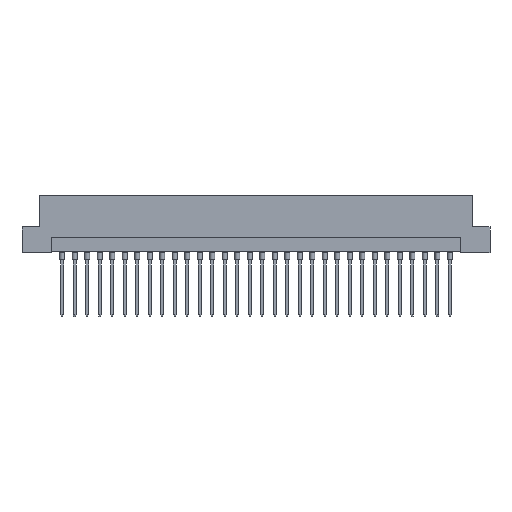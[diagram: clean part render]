
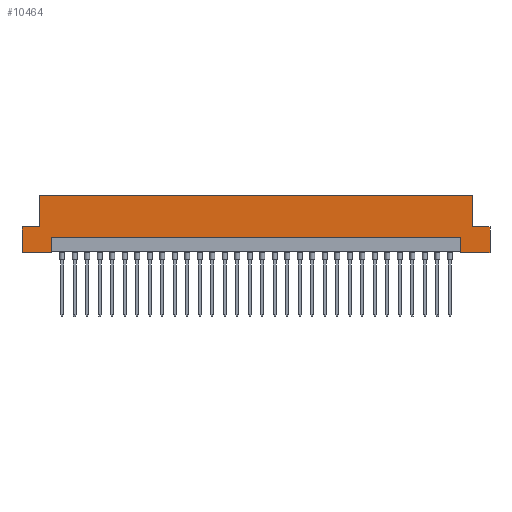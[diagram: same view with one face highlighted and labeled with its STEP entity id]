
A CAD part, front view. The second image highlights one B-rep face of the part: STEP entity #10464.
In plain terms, the highlighted planar face has unit normal (0, -1, 0).
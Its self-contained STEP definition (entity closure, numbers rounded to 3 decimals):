
#537 = CARTESIAN_POINT ( 'NONE',  ( -41.6, -4.3, 0. ) ) ;
#689 = ORIENTED_EDGE ( 'NONE', *, *, #5636, .F. ) ;
#698 = EDGE_CURVE ( 'NONE', #7802, #4916, #2948, .T. ) ;
#783 = DIRECTION ( 'NONE',  ( 1., 0., 0. ) ) ;
#962 = LINE ( 'NONE', #6274, #11961 ) ;
#1484 = ORIENTED_EDGE ( 'NONE', *, *, #698, .F. ) ;
#1489 = VECTOR ( 'NONE', #2459, 1000. ) ;
#1511 = VECTOR ( 'NONE', #783, 1000. ) ;
#1996 = CARTESIAN_POINT ( 'NONE',  ( 47.5, -4.3, 0. ) ) ;
#2158 = DIRECTION ( 'NONE',  ( 1., 0., 0. ) ) ;
#2159 = EDGE_CURVE ( 'NONE', #3640, #11440, #4019, .T. ) ;
#2447 = VECTOR ( 'NONE', #13092, 1000. ) ;
#2459 = DIRECTION ( 'NONE',  ( 1., 0., 0. ) ) ;
#2513 = LINE ( 'NONE', #3584, #10403 ) ;
#2587 = VECTOR ( 'NONE', #7142, 1000. ) ;
#2603 = LINE ( 'NONE', #9913, #11557 ) ;
#2709 = ORIENTED_EDGE ( 'NONE', *, *, #9408, .T. ) ;
#2948 = LINE ( 'NONE', #4141, #6473 ) ;
#3002 = CARTESIAN_POINT ( 'NONE',  ( -47.5, -4.3, 5.2 ) ) ;
#3094 = DIRECTION ( 'NONE',  ( 0., 0., -1. ) ) ;
#3239 = ORIENTED_EDGE ( 'NONE', *, *, #9156, .F. ) ;
#3276 = EDGE_CURVE ( 'NONE', #5323, #5963, #2603, .T. ) ;
#3437 = CARTESIAN_POINT ( 'NONE',  ( 41.6, -4.3, 0. ) ) ;
#3564 = EDGE_CURVE ( 'NONE', #6624, #9732, #5309, .T. ) ;
#3584 = CARTESIAN_POINT ( 'NONE',  ( 41.6, -4.3, 0.2 ) ) ;
#3640 = VERTEX_POINT ( 'NONE', #3437 ) ;
#3717 = CARTESIAN_POINT ( 'NONE',  ( 47.5, -4.3, 11.6 ) ) ;
#3839 = ORIENTED_EDGE ( 'NONE', *, *, #3902, .T. ) ;
#3902 = EDGE_CURVE ( 'NONE', #11890, #5963, #6824, .T. ) ;
#3930 = CARTESIAN_POINT ( 'NONE',  ( 47.5, -4.3, 5.2 ) ) ;
#4019 = LINE ( 'NONE', #11302, #8169 ) ;
#4032 = DIRECTION ( 'NONE',  ( -1., 0., 0. ) ) ;
#4141 = CARTESIAN_POINT ( 'NONE',  ( -44., -4.3, 5.2 ) ) ;
#4298 = ORIENTED_EDGE ( 'NONE', *, *, #5062, .F. ) ;
#4318 = CARTESIAN_POINT ( 'NONE',  ( 47.5, -4.3, 11.6 ) ) ;
#4456 = VECTOR ( 'NONE', #2158, 1000. ) ;
#4537 = AXIS2_PLACEMENT_3D ( 'NONE', #3717, #6079, #4032 ) ;
#4629 = CARTESIAN_POINT ( 'NONE',  ( 41.6, -4.3, 3. ) ) ;
#4786 = EDGE_CURVE ( 'NONE', #5323, #8736, #12894, .T. ) ;
#4810 = LINE ( 'NONE', #8719, #12596 ) ;
#4916 = VERTEX_POINT ( 'NONE', #7189 ) ;
#4926 = VERTEX_POINT ( 'NONE', #3002 ) ;
#5013 = CARTESIAN_POINT ( 'NONE',  ( 44., -4.3, 5.2 ) ) ;
#5062 = EDGE_CURVE ( 'NONE', #4916, #9787, #8495, .T. ) ;
#5309 = LINE ( 'NONE', #3930, #2447 ) ;
#5323 = VERTEX_POINT ( 'NONE', #13076 ) ;
#5636 = EDGE_CURVE ( 'NONE', #3640, #8736, #2513, .T. ) ;
#5833 = EDGE_CURVE ( 'NONE', #4926, #7802, #9187, .T. ) ;
#5963 = VERTEX_POINT ( 'NONE', #537 ) ;
#6079 = DIRECTION ( 'NONE',  ( 0., 1., 0. ) ) ;
#6274 = CARTESIAN_POINT ( 'NONE',  ( 47.5, -4.3, 11.6 ) ) ;
#6473 = VECTOR ( 'NONE', #11171, 1000. ) ;
#6521 = CARTESIAN_POINT ( 'NONE',  ( 44., -4.3, 11.6 ) ) ;
#6624 = VERTEX_POINT ( 'NONE', #7639 ) ;
#6824 = LINE ( 'NONE', #10874, #1511 ) ;
#6860 = CARTESIAN_POINT ( 'NONE',  ( -41.6, -4.3, 3. ) ) ;
#7142 = DIRECTION ( 'NONE',  ( 0., 0., 1. ) ) ;
#7189 = CARTESIAN_POINT ( 'NONE',  ( -44., -4.3, 11.6 ) ) ;
#7532 = ORIENTED_EDGE ( 'NONE', *, *, #2159, .T. ) ;
#7557 = EDGE_CURVE ( 'NONE', #6624, #9787, #8068, .T. ) ;
#7623 = DIRECTION ( 'NONE',  ( 0., 0., 1. ) ) ;
#7639 = CARTESIAN_POINT ( 'NONE',  ( 44., -4.3, 5.2 ) ) ;
#7649 = DIRECTION ( 'NONE',  ( 0., 0., -1. ) ) ;
#7802 = VERTEX_POINT ( 'NONE', #12959 ) ;
#8060 = DIRECTION ( 'NONE',  ( 1., 0., 0. ) ) ;
#8068 = LINE ( 'NONE', #5013, #2587 ) ;
#8169 = VECTOR ( 'NONE', #8060, 1000. ) ;
#8199 = CARTESIAN_POINT ( 'NONE',  ( -47.5, -4.3, 5.2 ) ) ;
#8495 = LINE ( 'NONE', #4318, #1489 ) ;
#8719 = CARTESIAN_POINT ( 'NONE',  ( -47.5, -4.3, 11.6 ) ) ;
#8736 = VERTEX_POINT ( 'NONE', #4629 ) ;
#8900 = VECTOR ( 'NONE', #10782, 1000. ) ;
#9156 = EDGE_CURVE ( 'NONE', #9732, #11440, #962, .T. ) ;
#9187 = LINE ( 'NONE', #8199, #4456 ) ;
#9408 = EDGE_CURVE ( 'NONE', #4926, #11890, #4810, .T. ) ;
#9604 = ORIENTED_EDGE ( 'NONE', *, *, #7557, .T. ) ;
#9732 = VERTEX_POINT ( 'NONE', #11555 ) ;
#9787 = VERTEX_POINT ( 'NONE', #6521 ) ;
#9913 = CARTESIAN_POINT ( 'NONE',  ( -41.6, -4.3, 0.2 ) ) ;
#10064 = PLANE ( 'NONE',  #4537 ) ;
#10403 = VECTOR ( 'NONE', #7623, 1000. ) ;
#10464 = ADVANCED_FACE ( 'NONE', ( #12797 ), #10064, .F. ) ;
#10567 = ORIENTED_EDGE ( 'NONE', *, *, #3276, .F. ) ;
#10782 = DIRECTION ( 'NONE',  ( 1., 0., 0. ) ) ;
#10874 = CARTESIAN_POINT ( 'NONE',  ( 47.5, -4.3, 0. ) ) ;
#10958 = ORIENTED_EDGE ( 'NONE', *, *, #4786, .T. ) ;
#11171 = DIRECTION ( 'NONE',  ( 0., 0., 1. ) ) ;
#11302 = CARTESIAN_POINT ( 'NONE',  ( 47.5, -4.3, 0. ) ) ;
#11316 = ORIENTED_EDGE ( 'NONE', *, *, #3564, .F. ) ;
#11440 = VERTEX_POINT ( 'NONE', #1996 ) ;
#11555 = CARTESIAN_POINT ( 'NONE',  ( 47.5, -4.3, 5.2 ) ) ;
#11557 = VECTOR ( 'NONE', #7649, 1000. ) ;
#11870 = CARTESIAN_POINT ( 'NONE',  ( -47.5, -4.3, 0. ) ) ;
#11890 = VERTEX_POINT ( 'NONE', #11870 ) ;
#11953 = ORIENTED_EDGE ( 'NONE', *, *, #5833, .F. ) ;
#11961 = VECTOR ( 'NONE', #3094, 1000. ) ;
#12036 = DIRECTION ( 'NONE',  ( 0., 0., -1. ) ) ;
#12411 = EDGE_LOOP ( 'NONE', ( #10958, #689, #7532, #3239, #11316, #9604, #4298, #1484, #11953, #2709, #3839, #10567 ) ) ;
#12596 = VECTOR ( 'NONE', #12036, 1000. ) ;
#12797 = FACE_OUTER_BOUND ( 'NONE', #12411, .T. ) ;
#12894 = LINE ( 'NONE', #6860, #8900 ) ;
#12959 = CARTESIAN_POINT ( 'NONE',  ( -44., -4.3, 5.2 ) ) ;
#13076 = CARTESIAN_POINT ( 'NONE',  ( -41.6, -4.3, 3. ) ) ;
#13092 = DIRECTION ( 'NONE',  ( 1., 0., 0. ) ) ;
